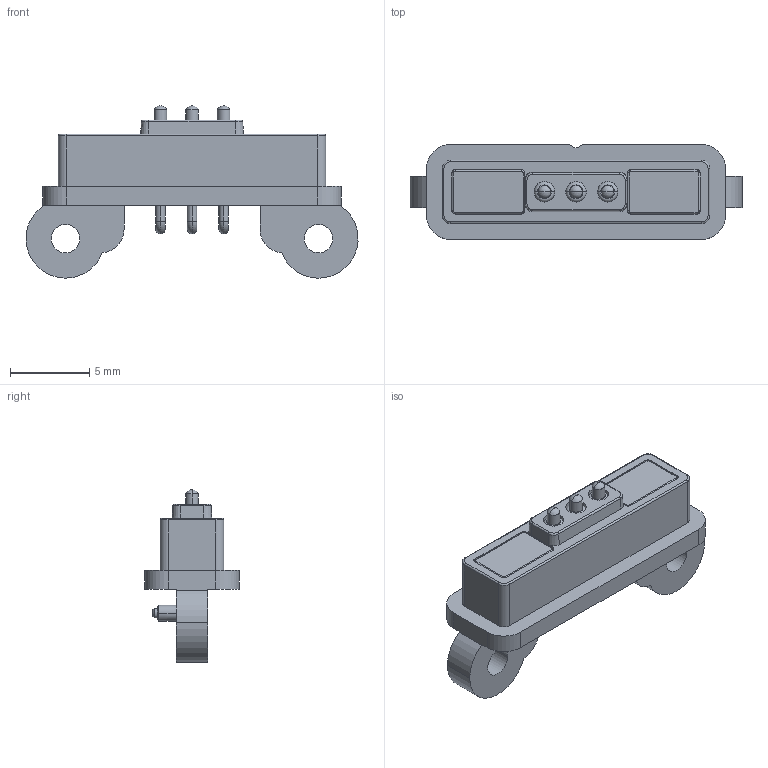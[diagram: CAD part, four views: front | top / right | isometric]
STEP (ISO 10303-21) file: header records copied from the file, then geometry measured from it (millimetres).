
FILE_DESCRIPTION (( 'STEP AP203' ), '1' );
FILE_NAME ('685-F0321351124.STEP', '2023-02-14T05:46:40', ( 'Magnum' ), ( '' ), 'SwSTEP 2.0', 'SolidWorks 2020', '' );
FILE_SCHEMA (( 'CONFIG_CONTROL_DESIGN' ));
Length unit declared in the file: millimetre
Products named in the file (1): 685-F0321351124
Bounding box: 20.99 x 6 x 10.9 mm (x, y, z)
Volume: 426.3 mm3; surface area: 762.5 mm2
Topology: 1 solids, 6 shells, 251 faces, 570 edges, 348 vertices
Faces by surface type: cylinder 112, plane 75, torus 28, cone 22, bspline 8, sphere 6
Entity records: 7252 total; most frequent: CARTESIAN_POINT 1342, DIRECTION 1331, ORIENTED_EDGE 1140, EDGE_CURVE 570, AXIS2_PLACEMENT_3D 529, VERTEX_POINT 348, CIRCLE 285, EDGE_LOOP 282
